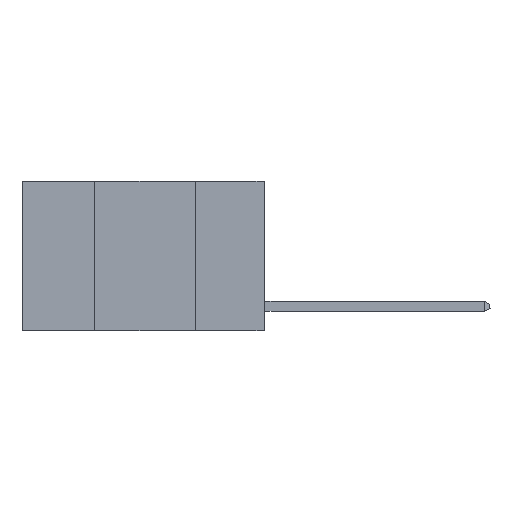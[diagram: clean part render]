
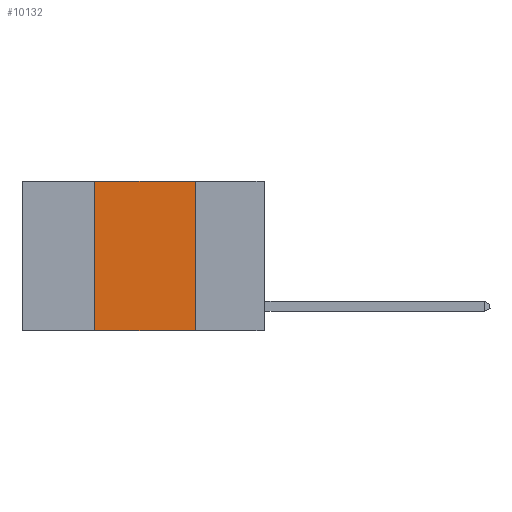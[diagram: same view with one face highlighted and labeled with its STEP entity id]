
A CAD part, left-side view. The second image highlights one B-rep face of the part: STEP entity #10132.
In plain terms, the highlighted planar face has unit normal (-1, 0, 0).
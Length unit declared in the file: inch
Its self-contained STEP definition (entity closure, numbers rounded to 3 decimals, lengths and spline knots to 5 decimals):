
#127 = DIRECTION ( 'NONE',  ( 1., 0., 0. ) ) ;
#1656 = VECTOR ( 'NONE', #5819, 39.37008 ) ;
#1948 = VECTOR ( 'NONE', #2945, 39.37008 ) ;
#2239 = ORIENTED_EDGE ( 'NONE', *, *, #10114, .F. ) ;
#2945 = DIRECTION ( 'NONE',  ( 0., -1., 0. ) ) ;
#5281 = VERTEX_POINT ( 'NONE', #16933 ) ;
#5510 = VECTOR ( 'NONE', #9498, 39.37008 ) ;
#5688 = FACE_OUTER_BOUND ( 'NONE', #12882, .T. ) ;
#5819 = DIRECTION ( 'NONE',  ( 0., 0., 1. ) ) ;
#6432 = VERTEX_POINT ( 'NONE', #14856 ) ;
#6636 = DIRECTION ( 'NONE',  ( 0., 0., -1. ) ) ;
#6722 = PLANE ( 'NONE',  #9544 ) ;
#6943 = CARTESIAN_POINT ( 'NONE',  ( 0., 0.42, 0. ) ) ;
#6994 = CARTESIAN_POINT ( 'NONE',  ( 0., 0.42, 0. ) ) ;
#8078 = VECTOR ( 'NONE', #10729, 39.37008 ) ;
#8602 = ORIENTED_EDGE ( 'NONE', *, *, #9835, .F. ) ;
#9498 = DIRECTION ( 'NONE',  ( 0., -1., 0. ) ) ;
#9544 = AXIS2_PLACEMENT_3D ( 'NONE', #12028, #127, #6636 ) ;
#9835 = EDGE_CURVE ( 'NONE', #6432, #14858, #16179, .T. ) ;
#9851 = EDGE_CURVE ( 'NONE', #6432, #15147, #14862, .T. ) ;
#10114 = EDGE_CURVE ( 'NONE', #14858, #5281, #10892, .T. ) ;
#10132 = ADVANCED_FACE ( 'NONE', ( #5688 ), #6722, .F. ) ;
#10729 = DIRECTION ( 'NONE',  ( 0., 0., -1. ) ) ;
#10844 = CARTESIAN_POINT ( 'NONE',  ( 0., 0.6, -0.37 ) ) ;
#10892 = LINE ( 'NONE', #13251, #5510 ) ;
#11421 = CARTESIAN_POINT ( 'NONE',  ( 0., 0.17, -0.37 ) ) ;
#12028 = CARTESIAN_POINT ( 'NONE',  ( 0., 0.6, 0. ) ) ;
#12196 = ORIENTED_EDGE ( 'NONE', *, *, #17208, .F. ) ;
#12882 = EDGE_LOOP ( 'NONE', ( #12196, #2239, #8602, #14591 ) ) ;
#13251 = CARTESIAN_POINT ( 'NONE',  ( 0., 0.6, 0. ) ) ;
#14591 = ORIENTED_EDGE ( 'NONE', *, *, #9851, .T. ) ;
#14753 = LINE ( 'NONE', #14842, #8078 ) ;
#14842 = CARTESIAN_POINT ( 'NONE',  ( 0., 0.17, 0. ) ) ;
#14856 = CARTESIAN_POINT ( 'NONE',  ( 0., 0.42, -0.37 ) ) ;
#14858 = VERTEX_POINT ( 'NONE', #6994 ) ;
#14862 = LINE ( 'NONE', #10844, #1948 ) ;
#15147 = VERTEX_POINT ( 'NONE', #11421 ) ;
#16179 = LINE ( 'NONE', #6943, #1656 ) ;
#16933 = CARTESIAN_POINT ( 'NONE',  ( 0., 0.17, 0. ) ) ;
#17208 = EDGE_CURVE ( 'NONE', #5281, #15147, #14753, .T. ) ;
